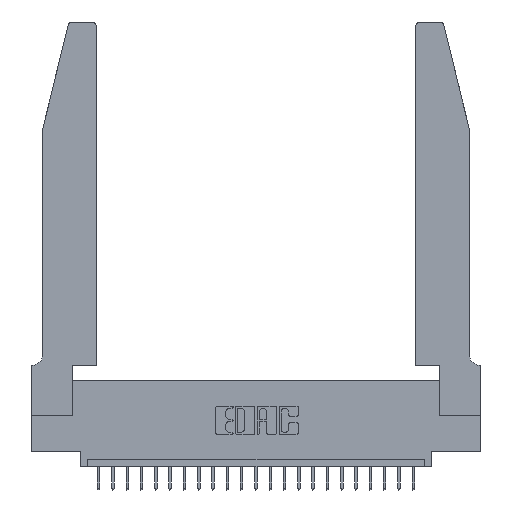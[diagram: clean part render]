
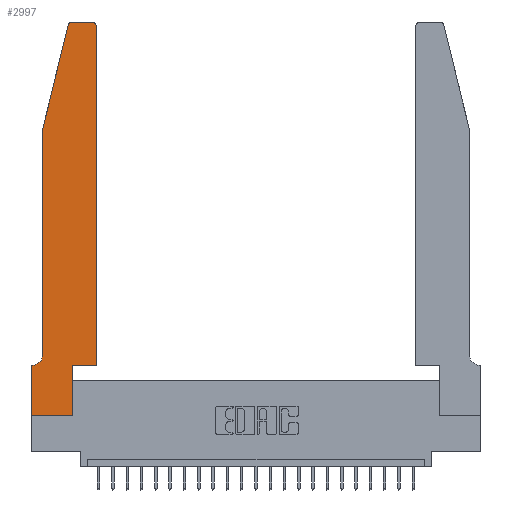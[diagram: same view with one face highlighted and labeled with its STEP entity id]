
A CAD part, top view. The second image highlights one B-rep face of the part: STEP entity #2997.
In plain terms, the highlighted planar face has unit normal (0, 0, 1).
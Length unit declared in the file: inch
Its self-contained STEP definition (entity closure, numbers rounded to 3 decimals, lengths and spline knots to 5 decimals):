
#12 = DIRECTION ( 'NONE',  ( 0., 1., 0. ) ) ;
#184 = EDGE_CURVE ( 'NONE', #13727, #24508, #19544, .T. ) ;
#623 = DIRECTION ( 'NONE',  ( 0., 0., 1. ) ) ;
#1037 = CARTESIAN_POINT ( 'NONE',  ( 0.4205, 2.72, 0.37 ) ) ;
#1622 = DIRECTION ( 'NONE',  ( -1., 0., 0. ) ) ;
#1676 = VECTOR ( 'NONE', #18575, 39.37008 ) ;
#2357 = DIRECTION ( 'NONE',  ( 1., 0., 0. ) ) ;
#2958 = CARTESIAN_POINT ( 'NONE',  ( 0.0755, 2., 0.37 ) ) ;
#2997 = ADVANCED_FACE ( 'NONE', ( #12207 ), #22962, .T. ) ;
#3049 = LINE ( 'NONE', #16967, #7898 ) ;
#3112 = VECTOR ( 'NONE', #4054, 39.37008 ) ;
#3114 = DIRECTION ( 'NONE',  ( 0., 0., 1. ) ) ;
#3791 = CARTESIAN_POINT ( 'NONE',  ( 0.2865, 0.35, 0.37 ) ) ;
#3848 = CARTESIAN_POINT ( 'NONE',  ( 0.0755, 0.42, 0.37 ) ) ;
#4054 = DIRECTION ( 'NONE',  ( -1., 0., 0. ) ) ;
#4677 = DIRECTION ( 'NONE',  ( 0., 0., -1. ) ) ;
#4707 = VERTEX_POINT ( 'NONE', #5755 ) ;
#4771 = EDGE_CURVE ( 'NONE', #16252, #8629, #11248, .T. ) ;
#4910 = CARTESIAN_POINT ( 'NONE',  ( 0.0755, 2., 0.37 ) ) ;
#5216 = EDGE_CURVE ( 'NONE', #24508, #4707, #14473, .T. ) ;
#5587 = CARTESIAN_POINT ( 'NONE',  ( 0.4505, 0.35, 0.37 ) ) ;
#5629 = LINE ( 'NONE', #14345, #9834 ) ;
#5755 = CARTESIAN_POINT ( 'NONE',  ( 0.4505, 0.35, 0.37 ) ) ;
#6085 = AXIS2_PLACEMENT_3D ( 'NONE', #8108, #623, #2357 ) ;
#6401 = ORIENTED_EDGE ( 'NONE', *, *, #184, .T. ) ;
#6736 = EDGE_LOOP ( 'NONE', ( #10801, #18302, #21557, #9882, #12729, #18592, #22588, #21805, #6401, #21902, #11664, #23921 ) ) ;
#7898 = VECTOR ( 'NONE', #13258, 39.37008 ) ;
#7997 = VERTEX_POINT ( 'NONE', #11336 ) ;
#8108 = CARTESIAN_POINT ( 'NONE',  ( 0.284, 2.72, 0.37 ) ) ;
#8449 = VECTOR ( 'NONE', #19385, 39.37008 ) ;
#8629 = VERTEX_POINT ( 'NONE', #13327 ) ;
#8778 = DIRECTION ( 'NONE',  ( 1., 0., 0. ) ) ;
#9395 = EDGE_CURVE ( 'NONE', #9736, #23901, #12306, .T. ) ;
#9577 = DIRECTION ( 'NONE',  ( 1., 0., 0. ) ) ;
#9736 = VERTEX_POINT ( 'NONE', #3848 ) ;
#9834 = VECTOR ( 'NONE', #22267, 39.37008 ) ;
#9882 = ORIENTED_EDGE ( 'NONE', *, *, #22735, .T. ) ;
#9922 = CARTESIAN_POINT ( 'NONE',  ( 0., 0.35, 0.37 ) ) ;
#10103 = CARTESIAN_POINT ( 'NONE',  ( 0., 0., 0.37 ) ) ;
#10533 = AXIS2_PLACEMENT_3D ( 'NONE', #19184, #15153, #9577 ) ;
#10801 = ORIENTED_EDGE ( 'NONE', *, *, #4771, .T. ) ;
#10869 = EDGE_CURVE ( 'NONE', #4707, #7997, #5629, .T. ) ;
#11224 = CARTESIAN_POINT ( 'NONE',  ( 0., 0., 0.37 ) ) ;
#11248 = LINE ( 'NONE', #19177, #3112 ) ;
#11266 = CARTESIAN_POINT ( 'NONE',  ( 0.4205, 2.75, 0.37 ) ) ;
#11336 = CARTESIAN_POINT ( 'NONE',  ( 0.4505, 2.72, 0.37 ) ) ;
#11664 = ORIENTED_EDGE ( 'NONE', *, *, #10869, .T. ) ;
#12207 = FACE_OUTER_BOUND ( 'NONE', #6736, .T. ) ;
#12211 = EDGE_CURVE ( 'NONE', #8629, #19409, #22379, .T. ) ;
#12245 = LINE ( 'NONE', #21017, #22167 ) ;
#12287 = EDGE_CURVE ( 'NONE', #7997, #16252, #21174, .T. ) ;
#12306 = CIRCLE ( 'NONE', #18644, 0.07 ) ;
#12330 = CARTESIAN_POINT ( 'NONE',  ( 0.0055, 0.42, 0.37 ) ) ;
#12567 = LINE ( 'NONE', #10103, #8449 ) ;
#12729 = ORIENTED_EDGE ( 'NONE', *, *, #9395, .T. ) ;
#12874 = DIRECTION ( 'NONE',  ( 0., -1., 0. ) ) ;
#13062 = VECTOR ( 'NONE', #12874, 39.37008 ) ;
#13258 = DIRECTION ( 'NONE',  ( -0.239, -0.971, 0. ) ) ;
#13327 = CARTESIAN_POINT ( 'NONE',  ( 0.284, 2.75, 0.37 ) ) ;
#13474 = VERTEX_POINT ( 'NONE', #4910 ) ;
#13727 = VERTEX_POINT ( 'NONE', #19374 ) ;
#14263 = LINE ( 'NONE', #11224, #13062 ) ;
#14345 = CARTESIAN_POINT ( 'NONE',  ( 0.4505, 0.35, 0.37 ) ) ;
#14408 = VECTOR ( 'NONE', #12, 39.37008 ) ;
#14473 = LINE ( 'NONE', #5587, #17196 ) ;
#14628 = VERTEX_POINT ( 'NONE', #15878 ) ;
#14839 = EDGE_CURVE ( 'NONE', #19409, #13474, #3049, .T. ) ;
#15153 = DIRECTION ( 'NONE',  ( 0., 0., 1. ) ) ;
#15878 = CARTESIAN_POINT ( 'NONE',  ( 0., 0., 0.37 ) ) ;
#16252 = VERTEX_POINT ( 'NONE', #11266 ) ;
#16367 = AXIS2_PLACEMENT_3D ( 'NONE', #1037, #3114, #8778 ) ;
#16967 = CARTESIAN_POINT ( 'NONE',  ( 0.0755, 2., 0.37 ) ) ;
#17196 = VECTOR ( 'NONE', #22944, 39.37008 ) ;
#17474 = CARTESIAN_POINT ( 'NONE',  ( 0.25487, 2.72718, 0.37 ) ) ;
#18302 = ORIENTED_EDGE ( 'NONE', *, *, #12211, .T. ) ;
#18575 = DIRECTION ( 'NONE',  ( 0., -1., 0. ) ) ;
#18592 = ORIENTED_EDGE ( 'NONE', *, *, #21312, .T. ) ;
#18644 = AXIS2_PLACEMENT_3D ( 'NONE', #12330, #4677, #23506 ) ;
#19177 = CARTESIAN_POINT ( 'NONE',  ( 0.2605, 2.75, 0.37 ) ) ;
#19184 = CARTESIAN_POINT ( 'NONE',  ( 0., 0.35, 0.37 ) ) ;
#19374 = CARTESIAN_POINT ( 'NONE',  ( 0.2865, 0., 0.37 ) ) ;
#19385 = DIRECTION ( 'NONE',  ( 1., 0., 0. ) ) ;
#19409 = VERTEX_POINT ( 'NONE', #17474 ) ;
#19544 = LINE ( 'NONE', #22958, #14408 ) ;
#20553 = CARTESIAN_POINT ( 'NONE',  ( 0.0055, 0.35, 0.37 ) ) ;
#20573 = EDGE_CURVE ( 'NONE', #14628, #13727, #12567, .T. ) ;
#20903 = LINE ( 'NONE', #2958, #1676 ) ;
#21017 = CARTESIAN_POINT ( 'NONE',  ( 0.0755, 0.35, 0.37 ) ) ;
#21174 = CIRCLE ( 'NONE', #16367, 0.03 ) ;
#21312 = EDGE_CURVE ( 'NONE', #23901, #23593, #12245, .T. ) ;
#21557 = ORIENTED_EDGE ( 'NONE', *, *, #14839, .T. ) ;
#21805 = ORIENTED_EDGE ( 'NONE', *, *, #20573, .T. ) ;
#21902 = ORIENTED_EDGE ( 'NONE', *, *, #5216, .T. ) ;
#22167 = VECTOR ( 'NONE', #1622, 39.37008 ) ;
#22231 = EDGE_CURVE ( 'NONE', #23593, #14628, #14263, .T. ) ;
#22267 = DIRECTION ( 'NONE',  ( 0., 1., 0. ) ) ;
#22379 = CIRCLE ( 'NONE', #6085, 0.03 ) ;
#22588 = ORIENTED_EDGE ( 'NONE', *, *, #22231, .T. ) ;
#22735 = EDGE_CURVE ( 'NONE', #13474, #9736, #20903, .T. ) ;
#22944 = DIRECTION ( 'NONE',  ( 1., 0., 0. ) ) ;
#22958 = CARTESIAN_POINT ( 'NONE',  ( 0.2865, 0.35, 0.37 ) ) ;
#22962 = PLANE ( 'NONE',  #10533 ) ;
#23506 = DIRECTION ( 'NONE',  ( -1., 0., 0. ) ) ;
#23593 = VERTEX_POINT ( 'NONE', #9922 ) ;
#23901 = VERTEX_POINT ( 'NONE', #20553 ) ;
#23921 = ORIENTED_EDGE ( 'NONE', *, *, #12287, .T. ) ;
#24508 = VERTEX_POINT ( 'NONE', #3791 ) ;
